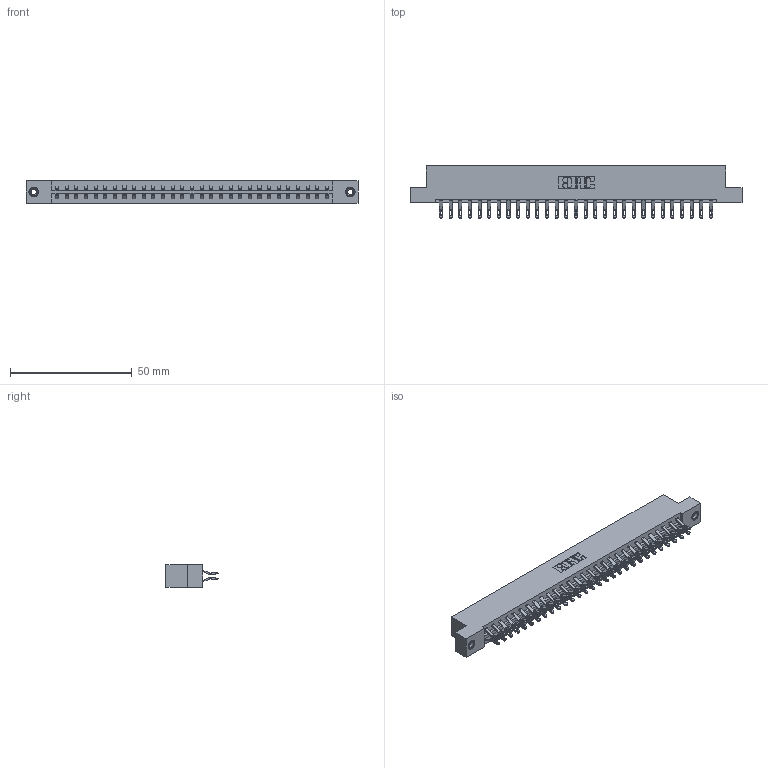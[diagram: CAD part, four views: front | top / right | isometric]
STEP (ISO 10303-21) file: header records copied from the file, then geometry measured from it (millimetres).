
FILE_DESCRIPTION (( 'STEP AP203' ), '1' );
FILE_NAME ('833-058-555-208.STEP', '2020-06-05T01:01:45', ( '' ), ( '' ), 'SwSTEP 2.0', 'SolidWorks 2020', '' );
FILE_SCHEMA (( 'CONFIG_CONTROL_DESIGN' ));
Length unit declared in the file: inch
Products named in the file (4): 833 Part_Flush - .156 Dia - TI; 345-292-001_555 Tail; 833-058-555-208; 345-250-001_345-250-003-102
Assembly tree (61 placements, depth 2):
  833-058-555-208
    833 Part_Flush - .156 Dia - TI
    345-292-001_555 Tail  x58
    345-250-001_345-250-003-102  x2
Bounding box: 136.45 x 21.47 x 9.4 mm (x, y, z)
Volume: 13970.8 mm3; surface area: 17028.2 mm2
Topology: 61 solids, 61 shells, 3538 faces, 11061 edges, 7366 vertices
Faces by surface type: plane 2074, cylinder 1448, cone 12, torus 4
Entity records: 21850 total; most frequent: CARTESIAN_POINT 3655, ORIENTED_EDGE 3554, DIRECTION 3147, EDGE_CURVE 1777, VECTOR 1609, LINE 1609, VERTEX_POINT 1180, AXIS2_PLACEMENT_3D 769
